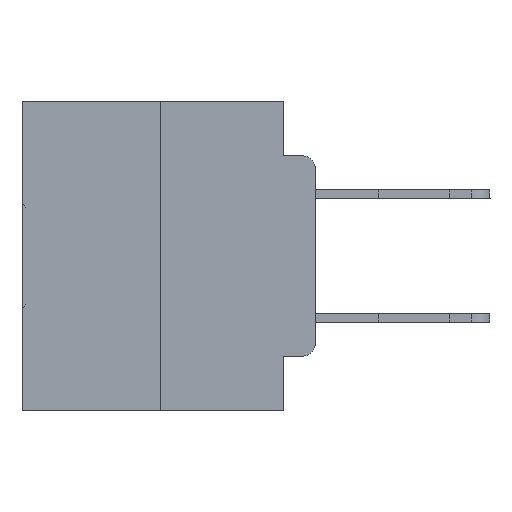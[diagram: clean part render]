
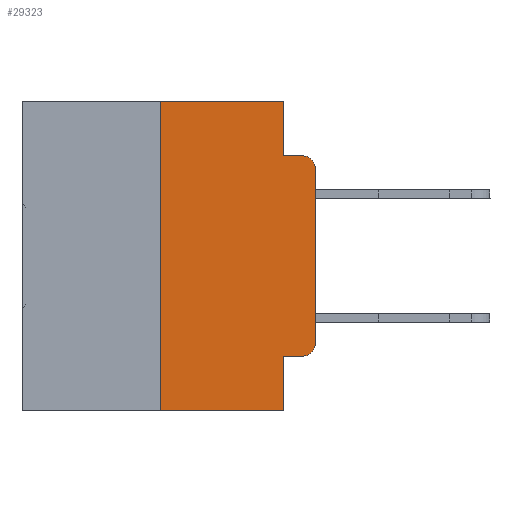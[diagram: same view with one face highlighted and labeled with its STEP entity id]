
A CAD part, left-side view. The second image highlights one B-rep face of the part: STEP entity #29323.
In plain terms, the highlighted planar face has unit normal (-1, 0, 0).
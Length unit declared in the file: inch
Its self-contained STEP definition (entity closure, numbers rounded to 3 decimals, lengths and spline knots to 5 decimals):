
#106 = ORIENTED_EDGE ( 'NONE', *, *, #23182, .T. ) ;
#749 = DIRECTION ( 'NONE',  ( 0., 0., -1. ) ) ;
#1043 = VERTEX_POINT ( 'NONE', #24410 ) ;
#1253 = DIRECTION ( 'NONE',  ( 0., -1., 0. ) ) ;
#1335 = CARTESIAN_POINT ( 'NONE',  ( 0., 0.02, -0.4115 ) ) ;
#1666 = ORIENTED_EDGE ( 'NONE', *, *, #9346, .T. ) ;
#1781 = LINE ( 'NONE', #11195, #14226 ) ;
#2083 = CARTESIAN_POINT ( 'NONE',  ( 0., 0.25, 0. ) ) ;
#2161 = VERTEX_POINT ( 'NONE', #2083 ) ;
#2292 = CARTESIAN_POINT ( 'NONE',  ( 0., 0.051, -0.0885 ) ) ;
#2498 = LINE ( 'NONE', #12359, #20610 ) ;
#2720 = EDGE_CURVE ( 'NONE', #30075, #8036, #12168, .T. ) ;
#3932 = DIRECTION ( 'NONE',  ( 0., 0., 1. ) ) ;
#4336 = LINE ( 'NONE', #18658, #23099 ) ;
#4401 = CARTESIAN_POINT ( 'NONE',  ( 0., 0.051, -0.4115 ) ) ;
#4758 = DIRECTION ( 'NONE',  ( 0., -1., 0. ) ) ;
#5629 = VECTOR ( 'NONE', #29875, 39.37008 ) ;
#6019 = EDGE_CURVE ( 'NONE', #30075, #31401, #29342, .T. ) ;
#6449 = ORIENTED_EDGE ( 'NONE', *, *, #27771, .F. ) ;
#6852 = PLANE ( 'NONE',  #8365 ) ;
#7492 = EDGE_CURVE ( 'NONE', #2161, #1043, #1781, .T. ) ;
#7582 = VECTOR ( 'NONE', #4758, 39.37008 ) ;
#7797 = VERTEX_POINT ( 'NONE', #12766 ) ;
#8036 = VERTEX_POINT ( 'NONE', #1335 ) ;
#8318 = DIRECTION ( 'NONE',  ( 0., 0., 1. ) ) ;
#8365 = AXIS2_PLACEMENT_3D ( 'NONE', #24007, #9418, #26398 ) ;
#9346 = EDGE_CURVE ( 'NONE', #9957, #16184, #4336, .T. ) ;
#9418 = DIRECTION ( 'NONE',  ( 1., 0., 0. ) ) ;
#9957 = VERTEX_POINT ( 'NONE', #20862 ) ;
#10436 = DIRECTION ( 'NONE',  ( -1., 0., 0. ) ) ;
#10701 = AXIS2_PLACEMENT_3D ( 'NONE', #24973, #10436, #27369 ) ;
#10824 = CARTESIAN_POINT ( 'NONE',  ( 0., 0.25, 0. ) ) ;
#11195 = CARTESIAN_POINT ( 'NONE',  ( 0., 0.473, 0. ) ) ;
#11449 = ORIENTED_EDGE ( 'NONE', *, *, #27849, .F. ) ;
#11700 = VECTOR ( 'NONE', #16067, 39.37008 ) ;
#11723 = DIRECTION ( 'NONE',  ( -1., 0., 0. ) ) ;
#12168 = LINE ( 'NONE', #4401, #5629 ) ;
#12359 = CARTESIAN_POINT ( 'NONE',  ( 0., 0.473, -0.5 ) ) ;
#12766 = CARTESIAN_POINT ( 'NONE',  ( 0., 0.02, -0.0885 ) ) ;
#12925 = CARTESIAN_POINT ( 'NONE',  ( 0., 0.051, -0.4115 ) ) ;
#13485 = AXIS2_PLACEMENT_3D ( 'NONE', #26229, #11723, #28579 ) ;
#14226 = VECTOR ( 'NONE', #1253, 39.37008 ) ;
#14271 = FACE_OUTER_BOUND ( 'NONE', #21629, .T. ) ;
#14420 = CARTESIAN_POINT ( 'NONE',  ( 0., 0., -0.1085 ) ) ;
#14626 = CARTESIAN_POINT ( 'NONE',  ( 0., 0.051, -0.5 ) ) ;
#14766 = VECTOR ( 'NONE', #8318, 39.37008 ) ;
#14838 = DIRECTION ( 'NONE',  ( 0., -1., 0. ) ) ;
#15645 = CARTESIAN_POINT ( 'NONE',  ( 0., 0.051, 0. ) ) ;
#16061 = ORIENTED_EDGE ( 'NONE', *, *, #31445, .T. ) ;
#16067 = DIRECTION ( 'NONE',  ( 0., 0., -1. ) ) ;
#16184 = VERTEX_POINT ( 'NONE', #14420 ) ;
#16801 = CIRCLE ( 'NONE', #10701, 0.02 ) ;
#18078 = EDGE_CURVE ( 'NONE', #31428, #7797, #26978, .T. ) ;
#18191 = LINE ( 'NONE', #25654, #11700 ) ;
#18658 = CARTESIAN_POINT ( 'NONE',  ( 0., 0., 0. ) ) ;
#19448 = CARTESIAN_POINT ( 'NONE',  ( 0., 0.25, -0.5 ) ) ;
#19465 = ORIENTED_EDGE ( 'NONE', *, *, #7492, .F. ) ;
#20610 = VECTOR ( 'NONE', #14838, 39.37008 ) ;
#20862 = CARTESIAN_POINT ( 'NONE',  ( 0., 0., -0.3915 ) ) ;
#20988 = CIRCLE ( 'NONE', #13485, 0.02 ) ;
#21629 = EDGE_LOOP ( 'NONE', ( #1666, #22088, #28919, #11449, #19465, #6449, #16061, #21737, #30719, #106 ) ) ;
#21737 = ORIENTED_EDGE ( 'NONE', *, *, #6019, .F. ) ;
#22088 = ORIENTED_EDGE ( 'NONE', *, *, #26055, .T. ) ;
#23068 = VECTOR ( 'NONE', #749, 39.37008 ) ;
#23099 = VECTOR ( 'NONE', #3932, 39.37008 ) ;
#23182 = EDGE_CURVE ( 'NONE', #8036, #9957, #16801, .T. ) ;
#24007 = CARTESIAN_POINT ( 'NONE',  ( 0., 0.473, 0. ) ) ;
#24410 = CARTESIAN_POINT ( 'NONE',  ( 0., 0.051, 0. ) ) ;
#24458 = CARTESIAN_POINT ( 'NONE',  ( 0., 0.051, -0.0885 ) ) ;
#24973 = CARTESIAN_POINT ( 'NONE',  ( 0., 0.02, -0.3915 ) ) ;
#25654 = CARTESIAN_POINT ( 'NONE',  ( 0., 0.051, 0. ) ) ;
#26055 = EDGE_CURVE ( 'NONE', #16184, #7797, #20988, .T. ) ;
#26229 = CARTESIAN_POINT ( 'NONE',  ( 0., 0.02, -0.1085 ) ) ;
#26398 = DIRECTION ( 'NONE',  ( 0., 0., -1. ) ) ;
#26978 = LINE ( 'NONE', #2292, #7582 ) ;
#27369 = DIRECTION ( 'NONE',  ( 0., 0., -1. ) ) ;
#27771 = EDGE_CURVE ( 'NONE', #30854, #2161, #28304, .T. ) ;
#27849 = EDGE_CURVE ( 'NONE', #1043, #31428, #18191, .T. ) ;
#28304 = LINE ( 'NONE', #10824, #14766 ) ;
#28579 = DIRECTION ( 'NONE',  ( 0., 0., -1. ) ) ;
#28919 = ORIENTED_EDGE ( 'NONE', *, *, #18078, .F. ) ;
#29323 = ADVANCED_FACE ( 'NONE', ( #14271 ), #6852, .F. ) ;
#29342 = LINE ( 'NONE', #15645, #23068 ) ;
#29875 = DIRECTION ( 'NONE',  ( 0., -1., 0. ) ) ;
#30075 = VERTEX_POINT ( 'NONE', #12925 ) ;
#30719 = ORIENTED_EDGE ( 'NONE', *, *, #2720, .T. ) ;
#30854 = VERTEX_POINT ( 'NONE', #19448 ) ;
#31401 = VERTEX_POINT ( 'NONE', #14626 ) ;
#31428 = VERTEX_POINT ( 'NONE', #24458 ) ;
#31445 = EDGE_CURVE ( 'NONE', #30854, #31401, #2498, .T. ) ;
